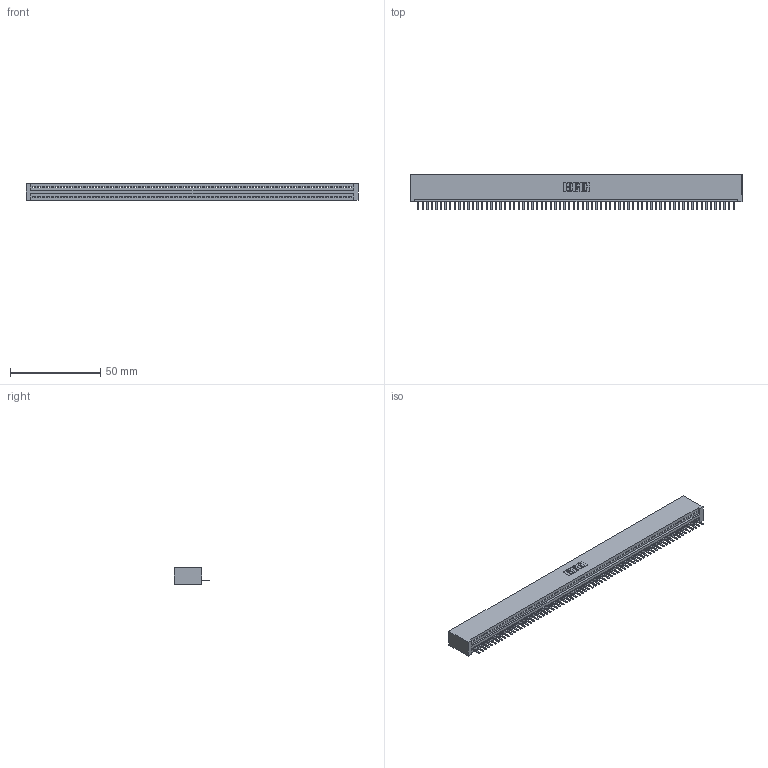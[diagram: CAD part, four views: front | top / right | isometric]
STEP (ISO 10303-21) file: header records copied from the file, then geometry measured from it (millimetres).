
FILE_DESCRIPTION (( 'STEP AP203' ), '1' );
FILE_NAME ('345-070-520-101.STEP', '2019-10-12T14:29:28', ( '' ), ( '' ), 'SwSTEP 2.0', 'SolidWorks 2016', '' );
FILE_SCHEMA (( 'CONFIG_CONTROL_DESIGN' ));
Length unit declared in the file: inch
Products named in the file (3): 345 Part_No Mounting Lugs; 345-070-520-101; 345-292-001_345-293-120
Assembly tree (71 placements, depth 2):
  345-070-520-101
    345 Part_No Mounting Lugs
    345-292-001_345-293-120  x70
Bounding box: 184.4 x 19.68 x 9.4 mm (x, y, z)
Volume: 18127.2 mm3; surface area: 24001.4 mm2
Topology: 71 solids, 71 shells, 4458 faces, 13197 edges, 8610 vertices
Faces by surface type: plane 3016, cylinder 1442
Entity records: 48751 total; most frequent: CARTESIAN_POINT 8462, ORIENTED_EDGE 8454, DIRECTION 7331, EDGE_CURVE 4227, LINE 3819, VECTOR 3819, VERTEX_POINT 2814, AXIS2_PLACEMENT_3D 1756
